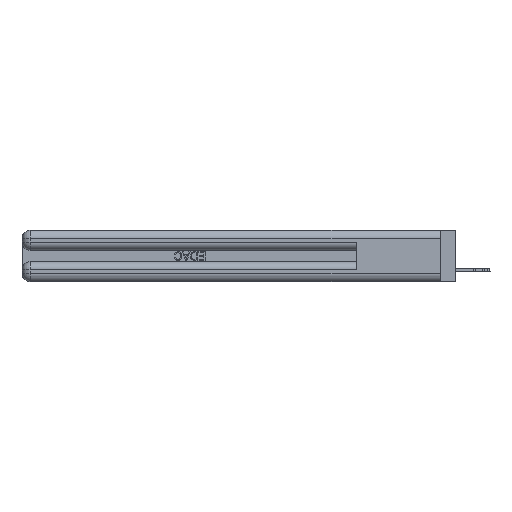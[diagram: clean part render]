
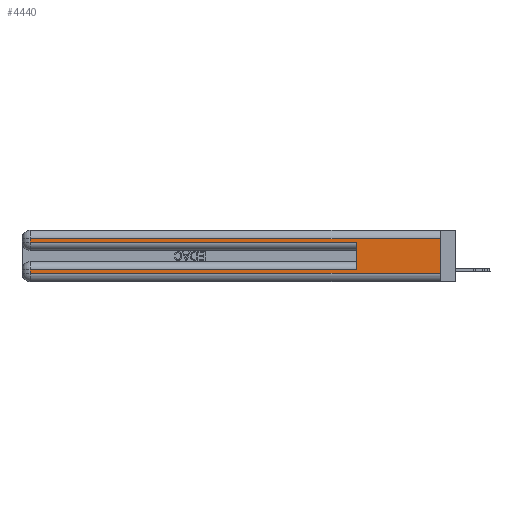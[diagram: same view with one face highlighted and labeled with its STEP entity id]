
A CAD part, left-side view. The second image highlights one B-rep face of the part: STEP entity #4440.
In plain terms, the highlighted planar face has unit normal (-1, 0, 0).
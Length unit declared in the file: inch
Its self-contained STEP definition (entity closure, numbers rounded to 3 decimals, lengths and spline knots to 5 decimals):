
#328 = CARTESIAN_POINT ( 'NONE',  ( 0., 2.94, 0.31 ) ) ;
#642 = EDGE_CURVE ( 'NONE', #16706, #1430, #9996, .T. ) ;
#1430 = VERTEX_POINT ( 'NONE', #17535 ) ;
#1935 = VECTOR ( 'NONE', #4988, 39.37008 ) ;
#2178 = VECTOR ( 'NONE', #38965, 39.37008 ) ;
#3781 = LINE ( 'NONE', #27600, #8579 ) ;
#4284 = CARTESIAN_POINT ( 'NONE',  ( 0., 0.6, 0.145 ) ) ;
#4401 = CARTESIAN_POINT ( 'NONE',  ( 0., 0., 0.31 ) ) ;
#4440 = ADVANCED_FACE ( 'NONE', ( #26171 ), #31076, .F. ) ;
#4951 = CARTESIAN_POINT ( 'NONE',  ( 0., 0., 0.37 ) ) ;
#4988 = DIRECTION ( 'NONE',  ( 0., -1., 0. ) ) ;
#6299 = ORIENTED_EDGE ( 'NONE', *, *, #18832, .T. ) ;
#7463 = DIRECTION ( 'NONE',  ( 0., 0., -1. ) ) ;
#8335 = ORIENTED_EDGE ( 'NONE', *, *, #12251, .F. ) ;
#8485 = VERTEX_POINT ( 'NONE', #16383 ) ;
#8579 = VECTOR ( 'NONE', #21093, 39.37008 ) ;
#8651 = CARTESIAN_POINT ( 'NONE',  ( 0., 2.94, 0.37 ) ) ;
#9395 = EDGE_CURVE ( 'NONE', #17203, #30323, #37458, .T. ) ;
#9996 = LINE ( 'NONE', #14098, #14720 ) ;
#10452 = VECTOR ( 'NONE', #31658, 39.37008 ) ;
#11833 = EDGE_CURVE ( 'NONE', #27971, #30323, #37745, .T. ) ;
#12060 = LINE ( 'NONE', #22701, #1935 ) ;
#12251 = EDGE_CURVE ( 'NONE', #16706, #41450, #43062, .T. ) ;
#13418 = ORIENTED_EDGE ( 'NONE', *, *, #9395, .F. ) ;
#13643 = ORIENTED_EDGE ( 'NONE', *, *, #23671, .T. ) ;
#14098 = CARTESIAN_POINT ( 'NONE',  ( 0., 0., 0.085 ) ) ;
#14720 = VECTOR ( 'NONE', #34498, 39.37008 ) ;
#16093 = CARTESIAN_POINT ( 'NONE',  ( 0., 0.6, 0.285 ) ) ;
#16383 = CARTESIAN_POINT ( 'NONE',  ( 0., 2.94, 0.285 ) ) ;
#16706 = VERTEX_POINT ( 'NONE', #42997 ) ;
#17001 = ORIENTED_EDGE ( 'NONE', *, *, #11833, .T. ) ;
#17158 = ORIENTED_EDGE ( 'NONE', *, *, #642, .T. ) ;
#17203 = VERTEX_POINT ( 'NONE', #23979 ) ;
#17432 = CARTESIAN_POINT ( 'NONE',  ( 0., 0., 0.37 ) ) ;
#17535 = CARTESIAN_POINT ( 'NONE',  ( 0., 2.94, 0.085 ) ) ;
#18460 = CARTESIAN_POINT ( 'NONE',  ( 0., 0., 0.06 ) ) ;
#18832 = EDGE_CURVE ( 'NONE', #17203, #33712, #43925, .T. ) ;
#21093 = DIRECTION ( 'NONE',  ( 0., 0., -1. ) ) ;
#21521 = AXIS2_PLACEMENT_3D ( 'NONE', #17432, #24406, #7463 ) ;
#21853 = DIRECTION ( 'NONE',  ( 0., 0., 1. ) ) ;
#22701 = CARTESIAN_POINT ( 'NONE',  ( 0., 0., 0.285 ) ) ;
#23671 = EDGE_CURVE ( 'NONE', #1430, #27971, #43528, .T. ) ;
#23979 = CARTESIAN_POINT ( 'NONE',  ( 0., 0., 0.31 ) ) ;
#24406 = DIRECTION ( 'NONE',  ( 1., 0., 0. ) ) ;
#26171 = FACE_OUTER_BOUND ( 'NONE', #34622, .T. ) ;
#26917 = VECTOR ( 'NONE', #32556, 39.37008 ) ;
#27600 = CARTESIAN_POINT ( 'NONE',  ( 0., 2.94, 0.37 ) ) ;
#27971 = VERTEX_POINT ( 'NONE', #29517 ) ;
#29517 = CARTESIAN_POINT ( 'NONE',  ( 0., 2.94, 0.06 ) ) ;
#30323 = VERTEX_POINT ( 'NONE', #30332 ) ;
#30332 = CARTESIAN_POINT ( 'NONE',  ( 0., 0., 0.06 ) ) ;
#31076 = PLANE ( 'NONE',  #21521 ) ;
#31205 = VECTOR ( 'NONE', #21853, 39.37008 ) ;
#31434 = ORIENTED_EDGE ( 'NONE', *, *, #37919, .T. ) ;
#31658 = DIRECTION ( 'NONE',  ( 0., -1., 0. ) ) ;
#32556 = DIRECTION ( 'NONE',  ( 0., 0., -1. ) ) ;
#33712 = VERTEX_POINT ( 'NONE', #328 ) ;
#34498 = DIRECTION ( 'NONE',  ( 0., 1., 0. ) ) ;
#34622 = EDGE_LOOP ( 'NONE', ( #13418, #6299, #31434, #41618, #8335, #17158, #13643, #17001 ) ) ;
#34872 = DIRECTION ( 'NONE',  ( 0., 1., 0. ) ) ;
#35859 = VECTOR ( 'NONE', #34872, 39.37008 ) ;
#37458 = LINE ( 'NONE', #4951, #2178 ) ;
#37745 = LINE ( 'NONE', #18460, #10452 ) ;
#37919 = EDGE_CURVE ( 'NONE', #33712, #8485, #3781, .T. ) ;
#38965 = DIRECTION ( 'NONE',  ( 0., 0., -1. ) ) ;
#40785 = EDGE_CURVE ( 'NONE', #8485, #41450, #12060, .T. ) ;
#41450 = VERTEX_POINT ( 'NONE', #16093 ) ;
#41618 = ORIENTED_EDGE ( 'NONE', *, *, #40785, .T. ) ;
#42997 = CARTESIAN_POINT ( 'NONE',  ( 0., 0.6, 0.085 ) ) ;
#43062 = LINE ( 'NONE', #4284, #31205 ) ;
#43528 = LINE ( 'NONE', #8651, #26917 ) ;
#43925 = LINE ( 'NONE', #4401, #35859 ) ;
